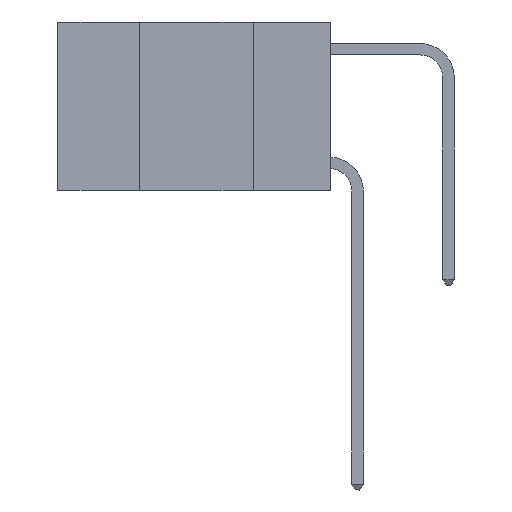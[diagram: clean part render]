
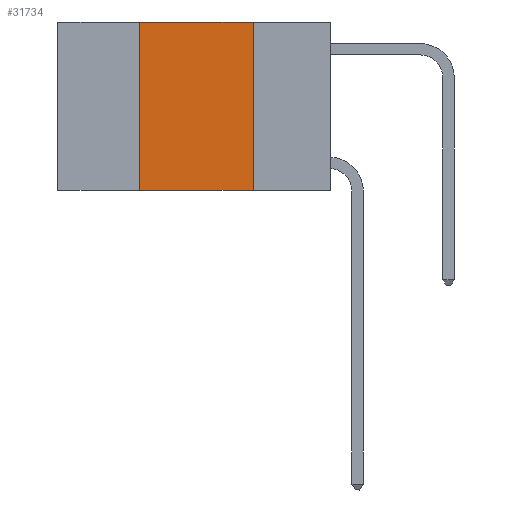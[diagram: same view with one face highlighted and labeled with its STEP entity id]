
A CAD part, left-side view. The second image highlights one B-rep face of the part: STEP entity #31734.
In plain terms, the highlighted planar face has unit normal (-1, 0, 0).
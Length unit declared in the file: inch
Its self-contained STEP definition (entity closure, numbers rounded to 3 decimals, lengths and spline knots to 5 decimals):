
#243 = DIRECTION ( 'NONE',  ( 0., -1., 0. ) ) ;
#1125 = ORIENTED_EDGE ( 'NONE', *, *, #8444, .F. ) ;
#2635 = VECTOR ( 'NONE', #10742, 39.37008 ) ;
#3613 = CARTESIAN_POINT ( 'NONE',  ( 0., 0.6, -0.37 ) ) ;
#4091 = VERTEX_POINT ( 'NONE', #27618 ) ;
#4207 = LINE ( 'NONE', #31343, #30997 ) ;
#5186 = EDGE_LOOP ( 'NONE', ( #23653, #1125, #27676, #17185 ) ) ;
#5878 = CARTESIAN_POINT ( 'NONE',  ( 0., 0.17, 0. ) ) ;
#6431 = DIRECTION ( 'NONE',  ( 0., 0., -1. ) ) ;
#7002 = LINE ( 'NONE', #21781, #14233 ) ;
#8444 = EDGE_CURVE ( 'NONE', #20544, #30213, #4207, .T. ) ;
#9541 = LINE ( 'NONE', #20365, #2635 ) ;
#10742 = DIRECTION ( 'NONE',  ( 0., 0., 1. ) ) ;
#12530 = DIRECTION ( 'NONE',  ( 1., 0., 0. ) ) ;
#14233 = VECTOR ( 'NONE', #6431, 39.37008 ) ;
#17185 = ORIENTED_EDGE ( 'NONE', *, *, #27744, .T. ) ;
#17604 = LINE ( 'NONE', #3613, #25251 ) ;
#19063 = FACE_OUTER_BOUND ( 'NONE', #5186, .T. ) ;
#20365 = CARTESIAN_POINT ( 'NONE',  ( 0., 0.42, 0. ) ) ;
#20488 = CARTESIAN_POINT ( 'NONE',  ( 0., 0.42, 0. ) ) ;
#20544 = VERTEX_POINT ( 'NONE', #20488 ) ;
#21768 = VERTEX_POINT ( 'NONE', #24271 ) ;
#21781 = CARTESIAN_POINT ( 'NONE',  ( 0., 0.17, 0. ) ) ;
#23236 = PLANE ( 'NONE',  #23911 ) ;
#23592 = EDGE_CURVE ( 'NONE', #21768, #20544, #9541, .T. ) ;
#23653 = ORIENTED_EDGE ( 'NONE', *, *, #24133, .F. ) ;
#23911 = AXIS2_PLACEMENT_3D ( 'NONE', #28191, #12530, #25525 ) ;
#24133 = EDGE_CURVE ( 'NONE', #30213, #4091, #7002, .T. ) ;
#24271 = CARTESIAN_POINT ( 'NONE',  ( 0., 0.42, -0.37 ) ) ;
#25251 = VECTOR ( 'NONE', #243, 39.37008 ) ;
#25525 = DIRECTION ( 'NONE',  ( 0., 0., -1. ) ) ;
#27618 = CARTESIAN_POINT ( 'NONE',  ( 0., 0.17, -0.37 ) ) ;
#27676 = ORIENTED_EDGE ( 'NONE', *, *, #23592, .F. ) ;
#27744 = EDGE_CURVE ( 'NONE', #21768, #4091, #17604, .T. ) ;
#28191 = CARTESIAN_POINT ( 'NONE',  ( 0., 0.6, 0. ) ) ;
#30213 = VERTEX_POINT ( 'NONE', #5878 ) ;
#30997 = VECTOR ( 'NONE', #31855, 39.37008 ) ;
#31343 = CARTESIAN_POINT ( 'NONE',  ( 0., 0.6, 0. ) ) ;
#31734 = ADVANCED_FACE ( 'NONE', ( #19063 ), #23236, .F. ) ;
#31855 = DIRECTION ( 'NONE',  ( 0., -1., 0. ) ) ;
